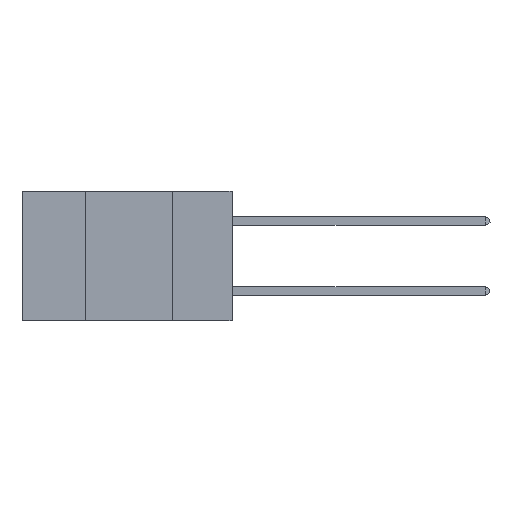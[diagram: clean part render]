
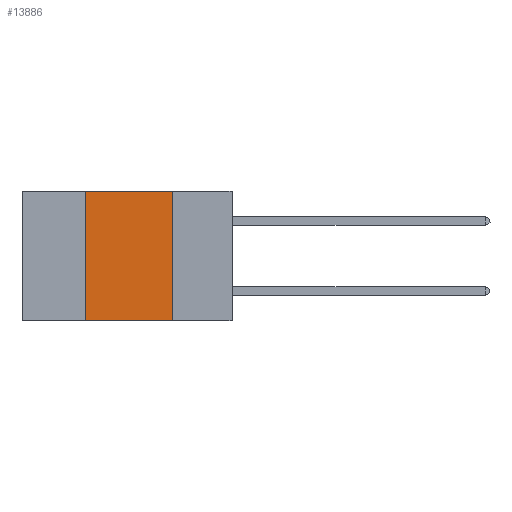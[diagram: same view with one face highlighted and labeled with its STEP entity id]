
A CAD part, left-side view. The second image highlights one B-rep face of the part: STEP entity #13886.
In plain terms, the highlighted planar face has unit normal (-1, 0, 0).
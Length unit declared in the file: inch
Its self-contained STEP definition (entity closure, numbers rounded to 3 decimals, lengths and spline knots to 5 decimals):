
#346 = VERTEX_POINT ( 'NONE', #8182 ) ;
#510 = DIRECTION ( 'NONE',  ( 1., 0., 0. ) ) ;
#670 = FACE_OUTER_BOUND ( 'NONE', #8324, .T. ) ;
#3161 = DIRECTION ( 'NONE',  ( 0., 0., -1. ) ) ;
#3194 = LINE ( 'NONE', #6938, #8331 ) ;
#3196 = DIRECTION ( 'NONE',  ( 0., -1., 0. ) ) ;
#3205 = ORIENTED_EDGE ( 'NONE', *, *, #11689, .T. ) ;
#3414 = ORIENTED_EDGE ( 'NONE', *, *, #10725, .F. ) ;
#3811 = CARTESIAN_POINT ( 'NONE',  ( 0., 0.17, 0. ) ) ;
#4742 = ORIENTED_EDGE ( 'NONE', *, *, #5711, .F. ) ;
#4835 = VERTEX_POINT ( 'NONE', #6304 ) ;
#5640 = VECTOR ( 'NONE', #3196, 39.37008 ) ;
#5650 = CARTESIAN_POINT ( 'NONE',  ( 0., 0.17, 0. ) ) ;
#5711 = EDGE_CURVE ( 'NONE', #13479, #9242, #8757, .T. ) ;
#5728 = VECTOR ( 'NONE', #6757, 39.37008 ) ;
#6304 = CARTESIAN_POINT ( 'NONE',  ( 0., 0.42, 0. ) ) ;
#6342 = DIRECTION ( 'NONE',  ( 0., 0., -1. ) ) ;
#6757 = DIRECTION ( 'NONE',  ( 0., 0., 1. ) ) ;
#6938 = CARTESIAN_POINT ( 'NONE',  ( 0., 0.6, 0. ) ) ;
#7207 = VECTOR ( 'NONE', #6342, 39.37008 ) ;
#7469 = ORIENTED_EDGE ( 'NONE', *, *, #9780, .F. ) ;
#8182 = CARTESIAN_POINT ( 'NONE',  ( 0., 0.42, -0.37 ) ) ;
#8324 = EDGE_LOOP ( 'NONE', ( #4742, #3414, #7469, #3205 ) ) ;
#8331 = VECTOR ( 'NONE', #11578, 39.37008 ) ;
#8757 = LINE ( 'NONE', #3811, #7207 ) ;
#9242 = VERTEX_POINT ( 'NONE', #12376 ) ;
#9274 = LINE ( 'NONE', #12865, #5640 ) ;
#9780 = EDGE_CURVE ( 'NONE', #346, #4835, #10283, .T. ) ;
#10283 = LINE ( 'NONE', #14117, #5728 ) ;
#10345 = PLANE ( 'NONE',  #15691 ) ;
#10725 = EDGE_CURVE ( 'NONE', #4835, #13479, #3194, .T. ) ;
#11578 = DIRECTION ( 'NONE',  ( 0., -1., 0. ) ) ;
#11689 = EDGE_CURVE ( 'NONE', #346, #9242, #9274, .T. ) ;
#12376 = CARTESIAN_POINT ( 'NONE',  ( 0., 0.17, -0.37 ) ) ;
#12865 = CARTESIAN_POINT ( 'NONE',  ( 0., 0.6, -0.37 ) ) ;
#13479 = VERTEX_POINT ( 'NONE', #5650 ) ;
#13886 = ADVANCED_FACE ( 'NONE', ( #670 ), #10345, .F. ) ;
#14117 = CARTESIAN_POINT ( 'NONE',  ( 0., 0.42, 0. ) ) ;
#15375 = CARTESIAN_POINT ( 'NONE',  ( 0., 0.6, 0. ) ) ;
#15691 = AXIS2_PLACEMENT_3D ( 'NONE', #15375, #510, #3161 ) ;
